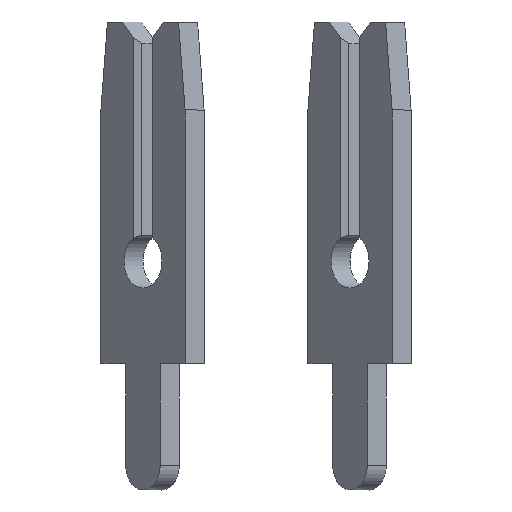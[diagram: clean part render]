
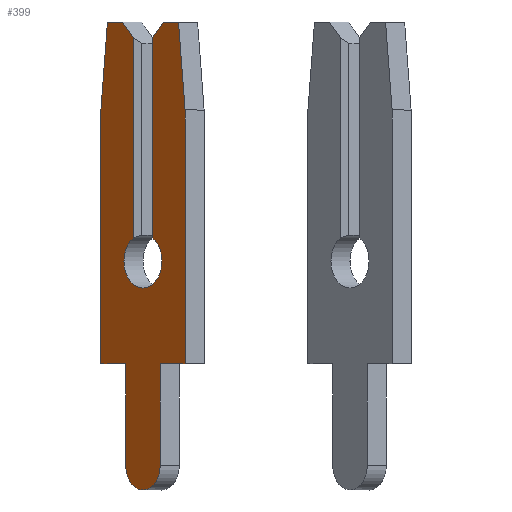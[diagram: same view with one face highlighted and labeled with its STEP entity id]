
A CAD part, top view. The second image highlights one B-rep face of the part: STEP entity #399.
In plain terms, the highlighted face is planar.
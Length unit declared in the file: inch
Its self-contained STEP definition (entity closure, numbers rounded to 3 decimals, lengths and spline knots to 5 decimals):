
#8 = CARTESIAN_POINT ( 'NONE',  ( -0.013, -0.1975, -0.0235 ) ) ;
#14 = DIRECTION ( 'NONE',  ( 0., 1., 0. ) ) ;
#18 = CARTESIAN_POINT ( 'NONE',  ( -0.013, 0.231, 0.028 ) ) ;
#20 = DIRECTION ( 'NONE',  ( 1., 0., 0. ) ) ;
#21 = LINE ( 'NONE', #1000, #606 ) ;
#43 = VECTOR ( 'NONE', #14, 39.37008 ) ;
#46 = DIRECTION ( 'NONE',  ( 0., 0., -1. ) ) ;
#51 = DIRECTION ( 'NONE',  ( 0., 0., -1. ) ) ;
#54 = DIRECTION ( 'NONE',  ( -1., 0., 0. ) ) ;
#59 = CARTESIAN_POINT ( 'NONE',  ( -0.013, -0.099, 0.0235 ) ) ;
#63 = CARTESIAN_POINT ( 'NONE',  ( -0.013, 0.231, 0.04857 ) ) ;
#74 = DIRECTION ( 'NONE',  ( 1., 0., 0. ) ) ;
#77 = VECTOR ( 'NONE', #925, 39.37008 ) ;
#81 = DIRECTION ( 'NONE',  ( 0., -1., 0. ) ) ;
#85 = VERTEX_POINT ( 'NONE', #763 ) ;
#86 = CARTESIAN_POINT ( 'NONE',  ( -0.013, 0.231, -0.04857 ) ) ;
#103 = CIRCLE ( 'NONE', #327, 0.026 ) ;
#105 = AXIS2_PLACEMENT_3D ( 'NONE', #837, #54, #827 ) ;
#114 = EDGE_CURVE ( 'NONE', #85, #125, #148, .T. ) ;
#123 = ORIENTED_EDGE ( 'NONE', *, *, #477, .F. ) ;
#125 = VERTEX_POINT ( 'NONE', #690 ) ;
#127 = LINE ( 'NONE', #951, #43 ) ;
#132 = CARTESIAN_POINT ( 'NONE',  ( -0.013, 0., 0. ) ) ;
#136 = VERTEX_POINT ( 'NONE', #989 ) ;
#147 = VECTOR ( 'NONE', #81, 39.37008 ) ;
#148 = LINE ( 'NONE', #59, #795 ) ;
#152 = CARTESIAN_POINT ( 'NONE',  ( -0.013, -0.099, 0.0575 ) ) ;
#153 = ORIENTED_EDGE ( 'NONE', *, *, #852, .F. ) ;
#154 = ORIENTED_EDGE ( 'NONE', *, *, #512, .T. ) ;
#163 = DIRECTION ( 'NONE',  ( 0., 0.995, 0.105 ) ) ;
#174 = ORIENTED_EDGE ( 'NONE', *, *, #839, .F. ) ;
#202 = VECTOR ( 'NONE', #711, 39.37008 ) ;
#208 = VECTOR ( 'NONE', #534, 39.37008 ) ;
#212 = ORIENTED_EDGE ( 'NONE', *, *, #565, .F. ) ;
#215 = LINE ( 'NONE', #843, #492 ) ;
#217 = DIRECTION ( 'NONE',  ( 0., -0.707, 0.707 ) ) ;
#220 = DIRECTION ( 'NONE',  ( 0., -1., 0. ) ) ;
#230 = VERTEX_POINT ( 'NONE', #290 ) ;
#245 = EDGE_CURVE ( 'NONE', #669, #490, #215, .T. ) ;
#250 = VERTEX_POINT ( 'NONE', #362 ) ;
#259 = DIRECTION ( 'NONE',  ( 0., 0., 1. ) ) ;
#264 = EDGE_CURVE ( 'NONE', #766, #774, #542, .T. ) ;
#277 = VECTOR ( 'NONE', #310, 39.37008 ) ;
#290 = CARTESIAN_POINT ( 'NONE',  ( -0.013, 0.02252, 0.013 ) ) ;
#298 = FACE_OUTER_BOUND ( 'NONE', #326, .T. ) ;
#310 = DIRECTION ( 'NONE',  ( 0., 1., 0. ) ) ;
#312 = VERTEX_POINT ( 'NONE', #615 ) ;
#321 = CARTESIAN_POINT ( 'NONE',  ( -0.013, 0.146, -0.0575 ) ) ;
#325 = CARTESIAN_POINT ( 'NONE',  ( -0.013, 0.231, -0.04857 ) ) ;
#326 = EDGE_LOOP ( 'NONE', ( #154, #153, #174, #560, #378, #415, #451, #858, #212, #507, #765, #374, #730, #802, #675, #437, #753, #123 ) ) ;
#327 = AXIS2_PLACEMENT_3D ( 'NONE', #132, #686, #46 ) ;
#335 = CARTESIAN_POINT ( 'NONE',  ( -0.013, 0.231, -0.028 ) ) ;
#340 = EDGE_CURVE ( 'NONE', #136, #965, #21, .T. ) ;
#350 = DIRECTION ( 'NONE',  ( -1., 0., 0. ) ) ;
#353 = CARTESIAN_POINT ( 'NONE',  ( -0.013, 0.146, 0.0575 ) ) ;
#357 = CIRCLE ( 'NONE', #105, 0.026 ) ;
#361 = LINE ( 'NONE', #401, #842 ) ;
#362 = CARTESIAN_POINT ( 'NONE',  ( -0.013, -0.099, 0.0575 ) ) ;
#374 = ORIENTED_EDGE ( 'NONE', *, *, #627, .F. ) ;
#378 = ORIENTED_EDGE ( 'NONE', *, *, #950, .F. ) ;
#387 = LINE ( 'NONE', #877, #147 ) ;
#395 = EDGE_CURVE ( 'NONE', #250, #85, #448, .T. ) ;
#399 = ADVANCED_FACE ( 'NONE', ( #298 ), #933, .F. ) ;
#401 = CARTESIAN_POINT ( 'NONE',  ( -0.013, 0.2105, 0.0075 ) ) ;
#415 = ORIENTED_EDGE ( 'NONE', *, *, #245, .F. ) ;
#431 = CARTESIAN_POINT ( 'NONE',  ( -0.013, 0.231, -0.028 ) ) ;
#433 = AXIS2_PLACEMENT_3D ( 'NONE', #667, #20, #259 ) ;
#437 = ORIENTED_EDGE ( 'NONE', *, *, #264, .F. ) ;
#448 = LINE ( 'NONE', #152, #208 ) ;
#451 = ORIENTED_EDGE ( 'NONE', *, *, #752, .F. ) ;
#453 = LINE ( 'NONE', #467, #202 ) ;
#454 = LINE ( 'NONE', #725, #277 ) ;
#467 = CARTESIAN_POINT ( 'NONE',  ( -0.013, 0., -0.013 ) ) ;
#477 = EDGE_CURVE ( 'NONE', #971, #987, #361, .T. ) ;
#486 = VERTEX_POINT ( 'NONE', #325 ) ;
#490 = VERTEX_POINT ( 'NONE', #881 ) ;
#492 = VECTOR ( 'NONE', #217, 39.37008 ) ;
#493 = CIRCLE ( 'NONE', #433, 0.0235 ) ;
#505 = VECTOR ( 'NONE', #513, 39.37008 ) ;
#506 = DIRECTION ( 'NONE',  ( 0., 0., 1. ) ) ;
#507 = ORIENTED_EDGE ( 'NONE', *, *, #340, .F. ) ;
#511 = VERTEX_POINT ( 'NONE', #321 ) ;
#512 = EDGE_CURVE ( 'NONE', #971, #230, #387, .T. ) ;
#513 = DIRECTION ( 'NONE',  ( 0., 0., 1. ) ) ;
#521 = EDGE_CURVE ( 'NONE', #592, #136, #454, .T. ) ;
#526 = CARTESIAN_POINT ( 'NONE',  ( -0.013, 0.146, 0.0575 ) ) ;
#533 = EDGE_CURVE ( 'NONE', #511, #486, #543, .T. ) ;
#534 = DIRECTION ( 'NONE',  ( 0., 0., -1. ) ) ;
#539 = CARTESIAN_POINT ( 'NONE',  ( -0.013, 0., 0. ) ) ;
#542 = LINE ( 'NONE', #63, #77 ) ;
#543 = LINE ( 'NONE', #86, #771 ) ;
#549 = VERTEX_POINT ( 'NONE', #556 ) ;
#556 = CARTESIAN_POINT ( 'NONE',  ( -0.013, 0., -0.026 ) ) ;
#560 = ORIENTED_EDGE ( 'NONE', *, *, #799, .F. ) ;
#565 = EDGE_CURVE ( 'NONE', #965, #511, #127, .T. ) ;
#588 = CARTESIAN_POINT ( 'NONE',  ( -0.013, 0.231, 0.04857 ) ) ;
#592 = VERTEX_POINT ( 'NONE', #8 ) ;
#602 = CARTESIAN_POINT ( 'NONE',  ( -0.013, 0.231, 0.028 ) ) ;
#606 = VECTOR ( 'NONE', #929, 39.37008 ) ;
#615 = CARTESIAN_POINT ( 'NONE',  ( -0.013, 0., 0.026 ) ) ;
#622 = LINE ( 'NONE', #431, #505 ) ;
#627 = EDGE_CURVE ( 'NONE', #125, #592, #493, .T. ) ;
#628 = DIRECTION ( 'NONE',  ( 0., 0., -1. ) ) ;
#636 = DIRECTION ( 'NONE',  ( 0., 0.707, 0.707 ) ) ;
#663 = CARTESIAN_POINT ( 'NONE',  ( -0.013, 0.02252, -0.013 ) ) ;
#667 = CARTESIAN_POINT ( 'NONE',  ( -0.013, -0.1975, 0. ) ) ;
#669 = VERTEX_POINT ( 'NONE', #335 ) ;
#673 = VERTEX_POINT ( 'NONE', #663 ) ;
#675 = ORIENTED_EDGE ( 'NONE', *, *, #906, .F. ) ;
#676 = VECTOR ( 'NONE', #506, 39.37008 ) ;
#686 = DIRECTION ( 'NONE',  ( -1., 0., 0. ) ) ;
#690 = CARTESIAN_POINT ( 'NONE',  ( -0.013, -0.1975, 0.0235 ) ) ;
#711 = DIRECTION ( 'NONE',  ( 0., -1., 0. ) ) ;
#725 = CARTESIAN_POINT ( 'NONE',  ( -0.013, -0.099, -0.0235 ) ) ;
#730 = ORIENTED_EDGE ( 'NONE', *, *, #114, .F. ) ;
#740 = EDGE_CURVE ( 'NONE', #987, #766, #876, .T. ) ;
#752 = EDGE_CURVE ( 'NONE', #486, #669, #622, .T. ) ;
#753 = ORIENTED_EDGE ( 'NONE', *, *, #740, .F. ) ;
#763 = CARTESIAN_POINT ( 'NONE',  ( -0.013, -0.099, 0.0235 ) ) ;
#765 = ORIENTED_EDGE ( 'NONE', *, *, #521, .F. ) ;
#766 = VERTEX_POINT ( 'NONE', #588 ) ;
#771 = VECTOR ( 'NONE', #163, 39.37008 ) ;
#774 = VERTEX_POINT ( 'NONE', #353 ) ;
#792 = VECTOR ( 'NONE', #986, 39.37008 ) ;
#795 = VECTOR ( 'NONE', #220, 39.37008 ) ;
#799 = EDGE_CURVE ( 'NONE', #673, #549, #979, .T. ) ;
#802 = ORIENTED_EDGE ( 'NONE', *, *, #395, .F. ) ;
#806 = CARTESIAN_POINT ( 'NONE',  ( -0.013, -0.099, -0.0575 ) ) ;
#811 = AXIS2_PLACEMENT_3D ( 'NONE', #976, #350, #51 ) ;
#827 = DIRECTION ( 'NONE',  ( 0., 0., -1. ) ) ;
#837 = CARTESIAN_POINT ( 'NONE',  ( -0.013, 0., 0. ) ) ;
#839 = EDGE_CURVE ( 'NONE', #549, #312, #357, .T. ) ;
#842 = VECTOR ( 'NONE', #636, 39.37008 ) ;
#843 = CARTESIAN_POINT ( 'NONE',  ( -0.013, 0.2105, -0.0075 ) ) ;
#852 = EDGE_CURVE ( 'NONE', #312, #230, #103, .T. ) ;
#858 = ORIENTED_EDGE ( 'NONE', *, *, #533, .F. ) ;
#876 = LINE ( 'NONE', #602, #676 ) ;
#877 = CARTESIAN_POINT ( 'NONE',  ( -0.013, 0.231, 0.013 ) ) ;
#881 = CARTESIAN_POINT ( 'NONE',  ( -0.013, 0.216, -0.013 ) ) ;
#882 = CARTESIAN_POINT ( 'NONE',  ( -0.013, 0.216, 0.013 ) ) ;
#891 = AXIS2_PLACEMENT_3D ( 'NONE', #539, #74, #628 ) ;
#906 = EDGE_CURVE ( 'NONE', #774, #250, #916, .T. ) ;
#916 = LINE ( 'NONE', #526, #792 ) ;
#925 = DIRECTION ( 'NONE',  ( 0., -0.995, 0.105 ) ) ;
#929 = DIRECTION ( 'NONE',  ( 0., 0., -1. ) ) ;
#933 = PLANE ( 'NONE',  #891 ) ;
#950 = EDGE_CURVE ( 'NONE', #490, #673, #453, .T. ) ;
#951 = CARTESIAN_POINT ( 'NONE',  ( -0.013, 0.146, -0.0575 ) ) ;
#965 = VERTEX_POINT ( 'NONE', #806 ) ;
#971 = VERTEX_POINT ( 'NONE', #882 ) ;
#976 = CARTESIAN_POINT ( 'NONE',  ( -0.013, 0., 0. ) ) ;
#979 = CIRCLE ( 'NONE', #811, 0.026 ) ;
#986 = DIRECTION ( 'NONE',  ( 0., -1., 0. ) ) ;
#987 = VERTEX_POINT ( 'NONE', #18 ) ;
#989 = CARTESIAN_POINT ( 'NONE',  ( -0.013, -0.099, -0.0235 ) ) ;
#1000 = CARTESIAN_POINT ( 'NONE',  ( -0.013, -0.099, -0.0575 ) ) ;
